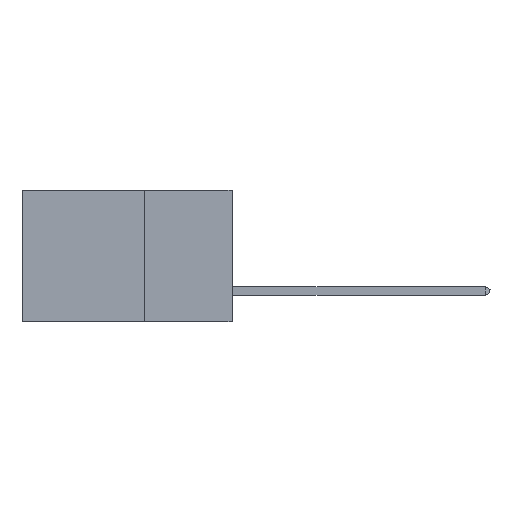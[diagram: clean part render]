
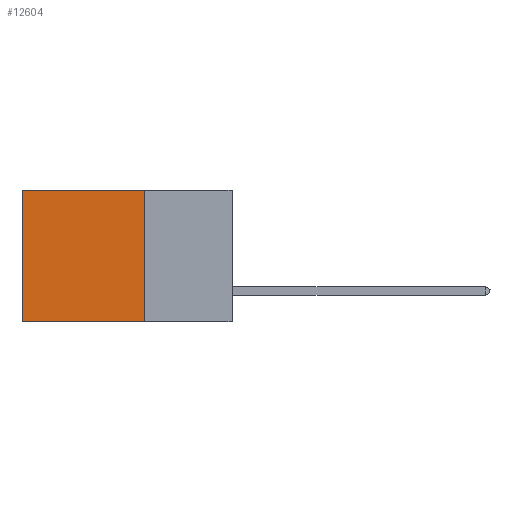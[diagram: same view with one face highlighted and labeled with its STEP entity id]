
A CAD part, left-side view. The second image highlights one B-rep face of the part: STEP entity #12604.
In plain terms, the highlighted planar face has unit normal (-1, 0, 0).
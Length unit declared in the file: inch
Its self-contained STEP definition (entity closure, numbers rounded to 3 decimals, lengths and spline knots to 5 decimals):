
#386 = PLANE ( 'NONE',  #719 ) ;
#446 = FACE_OUTER_BOUND ( 'NONE', #10099, .T. ) ;
#656 = VERTEX_POINT ( 'NONE', #5632 ) ;
#719 = AXIS2_PLACEMENT_3D ( 'NONE', #16615, #6880, #6228 ) ;
#1260 = DIRECTION ( 'NONE',  ( 0., 1., 0. ) ) ;
#2174 = EDGE_CURVE ( 'NONE', #14645, #19708, #2836, .T. ) ;
#2836 = LINE ( 'NONE', #18228, #20506 ) ;
#3341 = CARTESIAN_POINT ( 'NONE',  ( 0.2875, 0.25, 0. ) ) ;
#4301 = LINE ( 'NONE', #19190, #11156 ) ;
#4750 = EDGE_CURVE ( 'NONE', #12601, #656, #16423, .T. ) ;
#5632 = CARTESIAN_POINT ( 'NONE',  ( 0.2875, 0.25, -0.375 ) ) ;
#6228 = DIRECTION ( 'NONE',  ( 0., 0., -1. ) ) ;
#6880 = DIRECTION ( 'NONE',  ( 1., 0., 0. ) ) ;
#9252 = ORIENTED_EDGE ( 'NONE', *, *, #2174, .T. ) ;
#9424 = EDGE_CURVE ( 'NONE', #12601, #14645, #20255, .T. ) ;
#10099 = EDGE_LOOP ( 'NONE', ( #9252, #13054, #13116, #17889 ) ) ;
#10152 = DIRECTION ( 'NONE',  ( 0., 0., -1. ) ) ;
#11147 = EDGE_CURVE ( 'NONE', #656, #19708, #4301, .T. ) ;
#11156 = VECTOR ( 'NONE', #13203, 39.37008 ) ;
#12132 = VECTOR ( 'NONE', #17827, 39.37008 ) ;
#12601 = VERTEX_POINT ( 'NONE', #3341 ) ;
#12604 = ADVANCED_FACE ( 'NONE', ( #446 ), #386, .F. ) ;
#13054 = ORIENTED_EDGE ( 'NONE', *, *, #11147, .F. ) ;
#13116 = ORIENTED_EDGE ( 'NONE', *, *, #4750, .F. ) ;
#13203 = DIRECTION ( 'NONE',  ( 0., 1., 0. ) ) ;
#14645 = VERTEX_POINT ( 'NONE', #15011 ) ;
#14811 = CARTESIAN_POINT ( 'NONE',  ( 0.2875, 0.6, -0.375 ) ) ;
#15011 = CARTESIAN_POINT ( 'NONE',  ( 0.2875, 0.6, 0. ) ) ;
#16291 = CARTESIAN_POINT ( 'NONE',  ( 0.2875, 0.25, -0.375 ) ) ;
#16423 = LINE ( 'NONE', #16291, #12132 ) ;
#16615 = CARTESIAN_POINT ( 'NONE',  ( 0.2875, 0.25, -0.375 ) ) ;
#16985 = VECTOR ( 'NONE', #1260, 39.37008 ) ;
#17827 = DIRECTION ( 'NONE',  ( 0., 0., -1. ) ) ;
#17889 = ORIENTED_EDGE ( 'NONE', *, *, #9424, .T. ) ;
#18228 = CARTESIAN_POINT ( 'NONE',  ( 0.2875, 0.6, -0.375 ) ) ;
#19190 = CARTESIAN_POINT ( 'NONE',  ( 0.2875, 0.25, -0.375 ) ) ;
#19708 = VERTEX_POINT ( 'NONE', #14811 ) ;
#20255 = LINE ( 'NONE', #20719, #16985 ) ;
#20506 = VECTOR ( 'NONE', #10152, 39.37008 ) ;
#20719 = CARTESIAN_POINT ( 'NONE',  ( 0.2875, 0.25, 0. ) ) ;
